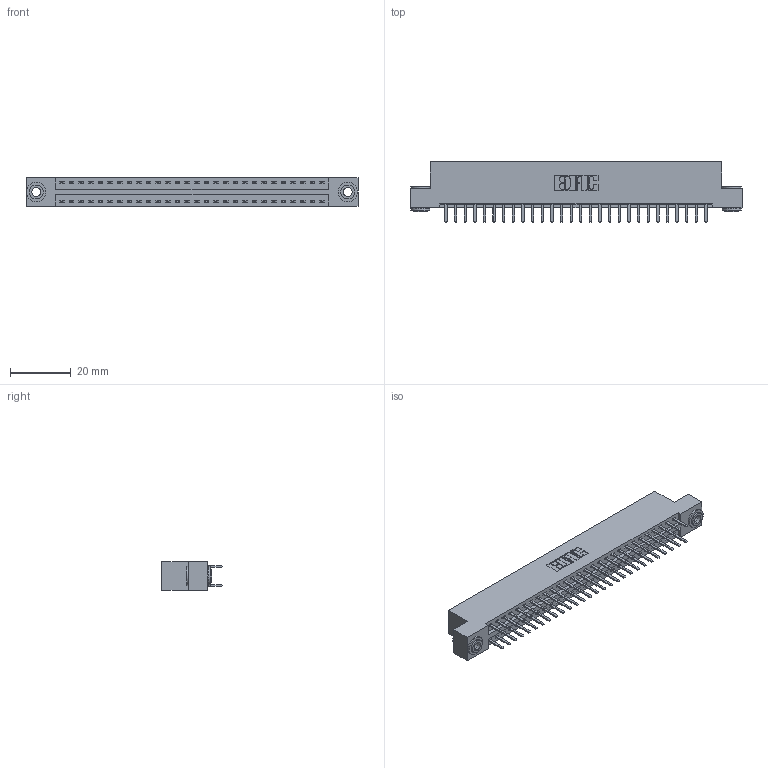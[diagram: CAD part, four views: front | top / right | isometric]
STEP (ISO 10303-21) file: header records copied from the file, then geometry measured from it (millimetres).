
FILE_DESCRIPTION (( 'STEP AP203' ), '1' );
FILE_NAME ('346-056-520-203.STEP', '2018-08-28T02:13:21', ( '' ), ( '' ), 'SwSTEP 2.0', 'SolidWorks 2016', '' );
FILE_SCHEMA (( 'CONFIG_CONTROL_DESIGN' ));
Length unit declared in the file: inch
Products named in the file (4): 345-250-002_345-250-002-102; 346-056-520-203; 346 Part_Flush Mounting Lugs - 0.156 Dia-TH; 345-292-001_345-293-120
Assembly tree (59 placements, depth 2):
  346-056-520-203
    346 Part_Flush Mounting Lugs - 0.156 Dia-TH
    345-292-001_345-293-120  x56
    345-250-002_345-250-002-102  x2
Bounding box: 109.47 x 20.02 x 9.4 mm (x, y, z)
Volume: 10561.1 mm3; surface area: 14453.4 mm2
Topology: 59 solids, 59 shells, 3296 faces, 9533 edges, 6202 vertices
Faces by surface type: plane 2158, cylinder 1130, cone 8
Entity records: 20922 total; most frequent: CARTESIAN_POINT 3455, ORIENTED_EDGE 3370, DIRECTION 3115, EDGE_CURVE 1685, LINE 1413, VECTOR 1413, VERTEX_POINT 1118, AXIS2_PLACEMENT_3D 851
